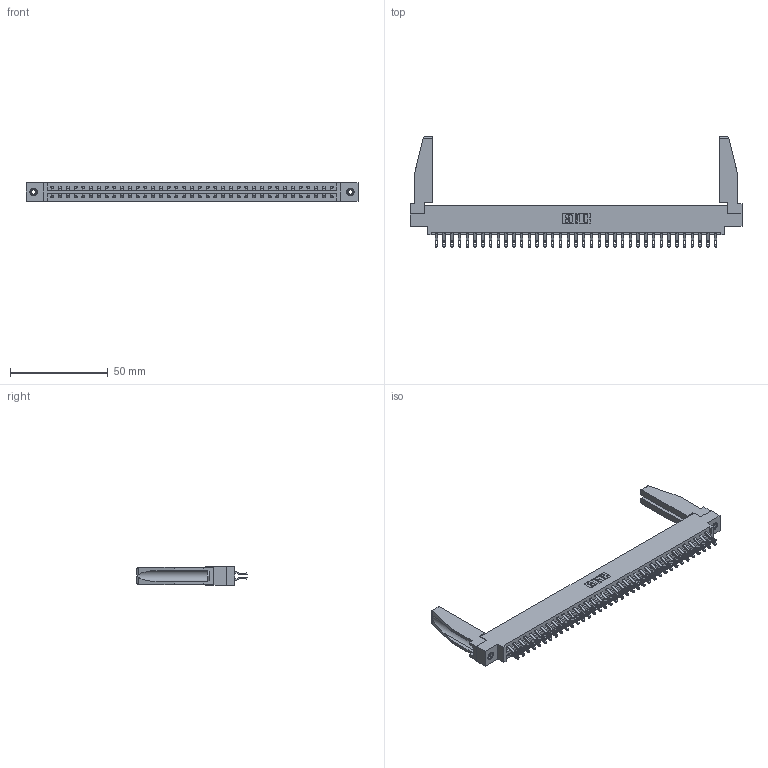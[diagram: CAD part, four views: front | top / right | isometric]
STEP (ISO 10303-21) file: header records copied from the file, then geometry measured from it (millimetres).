
FILE_DESCRIPTION (( 'STEP AP203' ), '1' );
FILE_NAME ('387-074-555-878.STEP', '2019-10-22T02:16:16', ( '' ), ( '' ), 'SwSTEP 2.0', 'SolidWorks 2016', '' );
FILE_SCHEMA (( 'CONFIG_CONTROL_DESIGN' ));
Length unit declared in the file: inch
Products named in the file (5): 387-074-555-878; 337 Part_0.170 Offset - 0.156 Dia-TI; 345-250-001_345-250-001-102; 307-220-078; 345-292-001_555 Tail
Assembly tree (79 placements, depth 2):
  387-074-555-878
    337 Part_0.170 Offset - 0.156 Dia-TI
    345-292-001_555 Tail  x74
    345-250-001_345-250-001-102  x2
    307-220-078  x2
Bounding box: 169.62 x 56.27 x 9.4 mm (x, y, z)
Volume: 21899.9 mm3; surface area: 24942.1 mm2
Topology: 79 solids, 79 shells, 4688 faces, 14639 edges, 9750 vertices
Faces by surface type: plane 2822, cylinder 1850, cone 12, torus 4
Entity records: 32232 total; most frequent: CARTESIAN_POINT 5470, ORIENTED_EDGE 5332, DIRECTION 4638, EDGE_CURVE 2666, LINE 2480, VECTOR 2480, VERTEX_POINT 1772, AXIS2_PLACEMENT_3D 1079
